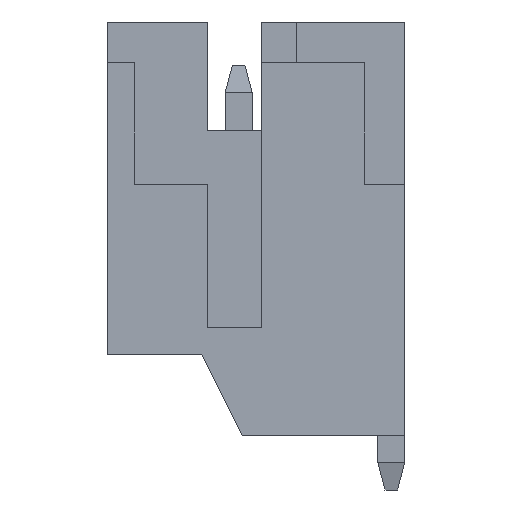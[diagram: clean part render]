
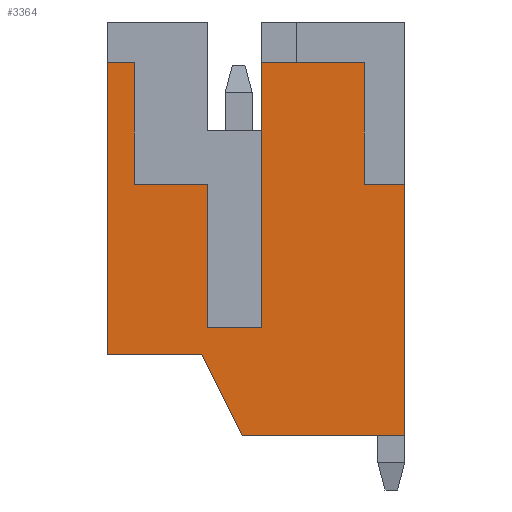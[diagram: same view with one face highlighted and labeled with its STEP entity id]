
A CAD part, left-side view. The second image highlights one B-rep face of the part: STEP entity #3364.
In plain terms, the highlighted planar face has unit normal (-1, 0, 0).
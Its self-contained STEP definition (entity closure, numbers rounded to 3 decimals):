
#27 = VECTOR ( 'NONE', #4020, 1000. ) ;
#160 = ORIENTED_EDGE ( 'NONE', *, *, #4919, .T. ) ;
#175 = VECTOR ( 'NONE', #6761, 1000. ) ;
#273 = CARTESIAN_POINT ( 'NONE',  ( -3., -2.32, 3.15 ) ) ;
#491 = EDGE_CURVE ( 'NONE', #8007, #7390, #2447, .T. ) ;
#526 = CARTESIAN_POINT ( 'NONE',  ( -3., 0.68, 0. ) ) ;
#535 = CARTESIAN_POINT ( 'NONE',  ( -3., 1.93, 5.4 ) ) ;
#730 = LINE ( 'NONE', #863, #4207 ) ;
#759 = VECTOR ( 'NONE', #6459, 1000. ) ;
#815 = CARTESIAN_POINT ( 'NONE',  ( -3., -0.07, -1.5 ) ) ;
#863 = CARTESIAN_POINT ( 'NONE',  ( -3., -0.42, 0.5 ) ) ;
#1035 = CARTESIAN_POINT ( 'NONE',  ( -3., -2.32, 3.15 ) ) ;
#1071 = EDGE_LOOP ( 'NONE', ( #2855, #8100, #6085, #8346, #6949, #1189, #7847, #160, #8911, #9094, #1774, #5853, #6087, #4442 ) ) ;
#1076 = DIRECTION ( 'NONE',  ( 0., 0., -1. ) ) ;
#1189 = ORIENTED_EDGE ( 'NONE', *, *, #4908, .T. ) ;
#1285 = CARTESIAN_POINT ( 'NONE',  ( -3., -3.07, -1.5 ) ) ;
#1395 = CARTESIAN_POINT ( 'NONE',  ( -3., 0., 0. ) ) ;
#1540 = EDGE_CURVE ( 'NONE', #4712, #5121, #730, .T. ) ;
#1561 = EDGE_CURVE ( 'NONE', #2098, #8987, #5533, .T. ) ;
#1602 = LINE ( 'NONE', #273, #7850 ) ;
#1624 = VECTOR ( 'NONE', #1076, 1000. ) ;
#1686 = LINE ( 'NONE', #7460, #4584 ) ;
#1774 = ORIENTED_EDGE ( 'NONE', *, *, #1540, .F. ) ;
#1784 = VERTEX_POINT ( 'NONE', #6487 ) ;
#1810 = DIRECTION ( 'NONE',  ( 0., -1., 0. ) ) ;
#1983 = CARTESIAN_POINT ( 'NONE',  ( -3., 2.43, 5.4 ) ) ;
#2031 = EDGE_CURVE ( 'NONE', #6602, #5098, #6531, .T. ) ;
#2034 = CARTESIAN_POINT ( 'NONE',  ( -3., -0.42, 5.4 ) ) ;
#2098 = VERTEX_POINT ( 'NONE', #4525 ) ;
#2284 = CARTESIAN_POINT ( 'NONE',  ( -3., 2.43, 0. ) ) ;
#2406 = VECTOR ( 'NONE', #7303, 1000. ) ;
#2409 = CARTESIAN_POINT ( 'NONE',  ( -3., -3.07, 5.4 ) ) ;
#2447 = LINE ( 'NONE', #815, #7359 ) ;
#2478 = VECTOR ( 'NONE', #3932, 1000. ) ;
#2646 = VERTEX_POINT ( 'NONE', #535 ) ;
#2745 = EDGE_CURVE ( 'NONE', #5098, #8007, #7759, .T. ) ;
#2855 = ORIENTED_EDGE ( 'NONE', *, *, #5671, .T. ) ;
#2858 = DIRECTION ( 'NONE',  ( 0., -0.447, -0.894 ) ) ;
#2926 = DIRECTION ( 'NONE',  ( 0., 0., -1. ) ) ;
#2957 = CARTESIAN_POINT ( 'NONE',  ( -3., -0.42, 6.15 ) ) ;
#3073 = VERTEX_POINT ( 'NONE', #2034 ) ;
#3228 = LINE ( 'NONE', #6508, #759 ) ;
#3364 = ADVANCED_FACE ( 'NONE', ( #8964 ), #3662, .T. ) ;
#3406 = DIRECTION ( 'NONE',  ( 0., -1., 0. ) ) ;
#3565 = DIRECTION ( 'NONE',  ( 0., -1., 0. ) ) ;
#3662 = PLANE ( 'NONE',  #4904 ) ;
#3677 = DIRECTION ( 'NONE',  ( 0., -1., 0. ) ) ;
#3736 = VERTEX_POINT ( 'NONE', #7113 ) ;
#3825 = CARTESIAN_POINT ( 'NONE',  ( -3., -0.07, -1.5 ) ) ;
#3932 = DIRECTION ( 'NONE',  ( 0., 1., 0. ) ) ;
#3944 = CARTESIAN_POINT ( 'NONE',  ( -3., 1.93, 3.15 ) ) ;
#3947 = EDGE_CURVE ( 'NONE', #3736, #4712, #5407, .T. ) ;
#3951 = VERTEX_POINT ( 'NONE', #3944 ) ;
#4020 = DIRECTION ( 'NONE',  ( 0., 0., 1. ) ) ;
#4046 = CARTESIAN_POINT ( 'NONE',  ( -3., -3.07, 6.15 ) ) ;
#4122 = VECTOR ( 'NONE', #2926, 1000. ) ;
#4189 = VERTEX_POINT ( 'NONE', #1285 ) ;
#4207 = VECTOR ( 'NONE', #1810, 1000. ) ;
#4441 = CARTESIAN_POINT ( 'NONE',  ( -3., -0.42, 3.15 ) ) ;
#4442 = ORIENTED_EDGE ( 'NONE', *, *, #7399, .T. ) ;
#4468 = CARTESIAN_POINT ( 'NONE',  ( -3., 2.43, 6.15 ) ) ;
#4483 = CARTESIAN_POINT ( 'NONE',  ( -3., -3.07, 3.15 ) ) ;
#4525 = CARTESIAN_POINT ( 'NONE',  ( -3., -2.32, 3.15 ) ) ;
#4584 = VECTOR ( 'NONE', #8908, 1000. ) ;
#4708 = DIRECTION ( 'NONE',  ( 0., 0., 1. ) ) ;
#4712 = VERTEX_POINT ( 'NONE', #8765 ) ;
#4904 = AXIS2_PLACEMENT_3D ( 'NONE', #1395, #7830, #3565 ) ;
#4908 = EDGE_CURVE ( 'NONE', #4189, #8987, #5958, .T. ) ;
#4919 = EDGE_CURVE ( 'NONE', #2098, #1784, #1602, .T. ) ;
#4981 = CARTESIAN_POINT ( 'NONE',  ( -3., -3.07, -1.5 ) ) ;
#5060 = CARTESIAN_POINT ( 'NONE',  ( -3., -0.42, 0.5 ) ) ;
#5098 = VERTEX_POINT ( 'NONE', #8693 ) ;
#5121 = VERTEX_POINT ( 'NONE', #5060 ) ;
#5357 = CARTESIAN_POINT ( 'NONE',  ( -3., 0.58, 3.15 ) ) ;
#5407 = LINE ( 'NONE', #5357, #1624 ) ;
#5467 = VECTOR ( 'NONE', #8529, 1000. ) ;
#5533 = LINE ( 'NONE', #1035, #175 ) ;
#5671 = EDGE_CURVE ( 'NONE', #2646, #6602, #7613, .T. ) ;
#5853 = ORIENTED_EDGE ( 'NONE', *, *, #3947, .F. ) ;
#5958 = LINE ( 'NONE', #4046, #27 ) ;
#6085 = ORIENTED_EDGE ( 'NONE', *, *, #2745, .T. ) ;
#6087 = ORIENTED_EDGE ( 'NONE', *, *, #8045, .F. ) ;
#6157 = LINE ( 'NONE', #4981, #5467 ) ;
#6459 = DIRECTION ( 'NONE',  ( 0., 1., 0. ) ) ;
#6487 = CARTESIAN_POINT ( 'NONE',  ( -3., -2.32, 5.4 ) ) ;
#6508 = CARTESIAN_POINT ( 'NONE',  ( -3., -3.07, 5.4 ) ) ;
#6531 = LINE ( 'NONE', #4468, #2406 ) ;
#6534 = VECTOR ( 'NONE', #3677, 1000. ) ;
#6602 = VERTEX_POINT ( 'NONE', #1983 ) ;
#6715 = EDGE_CURVE ( 'NONE', #7390, #4189, #6157, .T. ) ;
#6761 = DIRECTION ( 'NONE',  ( 0., -1., 0. ) ) ;
#6949 = ORIENTED_EDGE ( 'NONE', *, *, #6715, .T. ) ;
#7113 = CARTESIAN_POINT ( 'NONE',  ( -3., 0.58, 3.15 ) ) ;
#7303 = DIRECTION ( 'NONE',  ( 0., 0., -1. ) ) ;
#7359 = VECTOR ( 'NONE', #2858, 1000. ) ;
#7364 = LINE ( 'NONE', #4441, #8918 ) ;
#7390 = VERTEX_POINT ( 'NONE', #3825 ) ;
#7399 = EDGE_CURVE ( 'NONE', #3951, #2646, #1686, .T. ) ;
#7460 = CARTESIAN_POINT ( 'NONE',  ( -3., 1.93, 3.15 ) ) ;
#7613 = LINE ( 'NONE', #2409, #2478 ) ;
#7759 = LINE ( 'NONE', #2284, #6534 ) ;
#7769 = EDGE_CURVE ( 'NONE', #3073, #5121, #8150, .T. ) ;
#7830 = DIRECTION ( 'NONE',  ( -1., 0., 0. ) ) ;
#7847 = ORIENTED_EDGE ( 'NONE', *, *, #1561, .F. ) ;
#7850 = VECTOR ( 'NONE', #4708, 1000. ) ;
#8007 = VERTEX_POINT ( 'NONE', #526 ) ;
#8045 = EDGE_CURVE ( 'NONE', #3951, #3736, #7364, .T. ) ;
#8100 = ORIENTED_EDGE ( 'NONE', *, *, #2031, .T. ) ;
#8150 = LINE ( 'NONE', #2957, #4122 ) ;
#8270 = EDGE_CURVE ( 'NONE', #1784, #3073, #3228, .T. ) ;
#8346 = ORIENTED_EDGE ( 'NONE', *, *, #491, .T. ) ;
#8529 = DIRECTION ( 'NONE',  ( 0., -1., 0. ) ) ;
#8693 = CARTESIAN_POINT ( 'NONE',  ( -3., 2.43, 0. ) ) ;
#8765 = CARTESIAN_POINT ( 'NONE',  ( -3., 0.58, 0.5 ) ) ;
#8908 = DIRECTION ( 'NONE',  ( 0., 0., 1. ) ) ;
#8911 = ORIENTED_EDGE ( 'NONE', *, *, #8270, .T. ) ;
#8918 = VECTOR ( 'NONE', #3406, 1000. ) ;
#8964 = FACE_OUTER_BOUND ( 'NONE', #1071, .T. ) ;
#8987 = VERTEX_POINT ( 'NONE', #4483 ) ;
#9094 = ORIENTED_EDGE ( 'NONE', *, *, #7769, .T. ) ;
